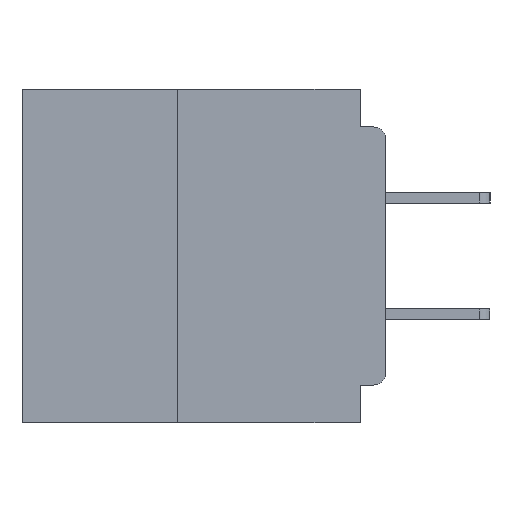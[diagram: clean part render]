
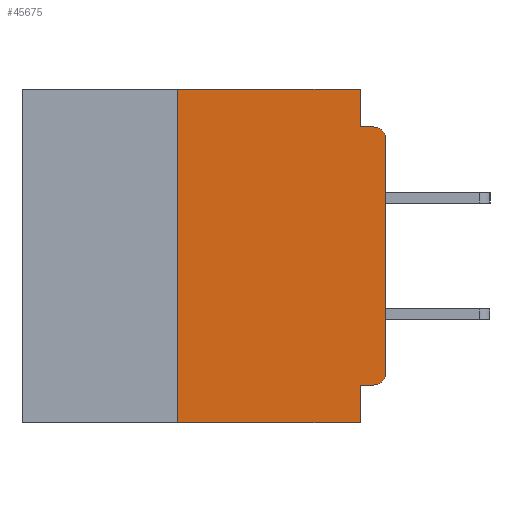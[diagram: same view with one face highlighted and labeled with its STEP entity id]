
A CAD part, left-side view. The second image highlights one B-rep face of the part: STEP entity #45675.
In plain terms, the highlighted planar face has unit normal (-1, 0, 0).
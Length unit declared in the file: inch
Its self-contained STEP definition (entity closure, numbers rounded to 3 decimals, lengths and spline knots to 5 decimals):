
#1313 = EDGE_CURVE ( 'NONE', #10483, #32483, #4898, .T. ) ;
#1629 = EDGE_CURVE ( 'NONE', #41125, #41036, #31239, .T. ) ;
#1631 = VERTEX_POINT ( 'NONE', #34603 ) ;
#1679 = ORIENTED_EDGE ( 'NONE', *, *, #33800, .F. ) ;
#1743 = CARTESIAN_POINT ( 'NONE',  ( 0., 0.031, 0. ) ) ;
#3261 = CARTESIAN_POINT ( 'NONE',  ( 0., 0.437, 0. ) ) ;
#3358 = ORIENTED_EDGE ( 'NONE', *, *, #36397, .F. ) ;
#4329 = CARTESIAN_POINT ( 'NONE',  ( 0., 0.437, 0. ) ) ;
#4350 = LINE ( 'NONE', #23653, #24455 ) ;
#4898 = LINE ( 'NONE', #48186, #14319 ) ;
#7079 = VECTOR ( 'NONE', #47031, 39.37008 ) ;
#7369 = LINE ( 'NONE', #23698, #26192 ) ;
#8332 = LINE ( 'NONE', #51061, #7079 ) ;
#8676 = CARTESIAN_POINT ( 'NONE',  ( 0., 0.015, -0.06 ) ) ;
#8730 = CARTESIAN_POINT ( 'NONE',  ( 0., 0.437, -0.4 ) ) ;
#10483 = VERTEX_POINT ( 'NONE', #18383 ) ;
#11990 = VECTOR ( 'NONE', #31342, 39.37008 ) ;
#12399 = PLANE ( 'NONE',  #33347 ) ;
#12697 = DIRECTION ( 'NONE',  ( 0., 0., -1. ) ) ;
#14319 = VECTOR ( 'NONE', #48076, 39.37008 ) ;
#14475 = CARTESIAN_POINT ( 'NONE',  ( 0., 0., 0. ) ) ;
#15382 = ORIENTED_EDGE ( 'NONE', *, *, #1629, .T. ) ;
#16089 = CARTESIAN_POINT ( 'NONE',  ( 0., 0.031, 0. ) ) ;
#16439 = DIRECTION ( 'NONE',  ( 0., 0., -1. ) ) ;
#16702 = CARTESIAN_POINT ( 'NONE',  ( 0., 0.031, -0.045 ) ) ;
#17888 = VECTOR ( 'NONE', #22523, 39.37008 ) ;
#18383 = CARTESIAN_POINT ( 'NONE',  ( 0., 0.25, -0.4 ) ) ;
#18413 = ORIENTED_EDGE ( 'NONE', *, *, #25655, .F. ) ;
#18552 = VERTEX_POINT ( 'NONE', #1743 ) ;
#19575 = CARTESIAN_POINT ( 'NONE',  ( 0., 0.25, 0. ) ) ;
#21410 = LINE ( 'NONE', #3261, #11990 ) ;
#21586 = ORIENTED_EDGE ( 'NONE', *, *, #1313, .F. ) ;
#22523 = DIRECTION ( 'NONE',  ( 0., 0., 1. ) ) ;
#23374 = VERTEX_POINT ( 'NONE', #36305 ) ;
#23653 = CARTESIAN_POINT ( 'NONE',  ( 0., 0.031, -0.4 ) ) ;
#23698 = CARTESIAN_POINT ( 'NONE',  ( 0., 0., -0.355 ) ) ;
#24372 = ORIENTED_EDGE ( 'NONE', *, *, #35073, .T. ) ;
#24425 = VECTOR ( 'NONE', #32782, 39.37008 ) ;
#24455 = VECTOR ( 'NONE', #27669, 39.37008 ) ;
#24699 = AXIS2_PLACEMENT_3D ( 'NONE', #33983, #33919, #33802 ) ;
#25389 = FACE_OUTER_BOUND ( 'NONE', #36045, .T. ) ;
#25655 = EDGE_CURVE ( 'NONE', #32483, #18552, #21410, .T. ) ;
#25910 = VECTOR ( 'NONE', #36122, 39.37008 ) ;
#26192 = VECTOR ( 'NONE', #47794, 39.37008 ) ;
#26659 = EDGE_CURVE ( 'NONE', #43019, #23374, #4350, .T. ) ;
#27158 = LINE ( 'NONE', #16089, #25910 ) ;
#27378 = AXIS2_PLACEMENT_3D ( 'NONE', #8676, #36779, #12697 ) ;
#27669 = DIRECTION ( 'NONE',  ( 0., 0., -1. ) ) ;
#27868 = CARTESIAN_POINT ( 'NONE',  ( 0., 0., -0.34 ) ) ;
#28113 = CARTESIAN_POINT ( 'NONE',  ( 0., 0., -0.06 ) ) ;
#30764 = ORIENTED_EDGE ( 'NONE', *, *, #49836, .T. ) ;
#31239 = CIRCLE ( 'NONE', #24699, 0.015 ) ;
#31342 = DIRECTION ( 'NONE',  ( 0., -1., 0. ) ) ;
#32483 = VERTEX_POINT ( 'NONE', #19575 ) ;
#32782 = DIRECTION ( 'NONE',  ( 0., -1., 0. ) ) ;
#33170 = CARTESIAN_POINT ( 'NONE',  ( 0., 0.031, -0.355 ) ) ;
#33347 = AXIS2_PLACEMENT_3D ( 'NONE', #4329, #40495, #16439 ) ;
#33800 = EDGE_CURVE ( 'NONE', #41125, #43019, #7369, .T. ) ;
#33802 = DIRECTION ( 'NONE',  ( 0., 0., -1. ) ) ;
#33849 = VERTEX_POINT ( 'NONE', #16702 ) ;
#33919 = DIRECTION ( 'NONE',  ( -1., 0., 0. ) ) ;
#33983 = CARTESIAN_POINT ( 'NONE',  ( 0., 0.015, -0.34 ) ) ;
#34603 = CARTESIAN_POINT ( 'NONE',  ( 0., 0.015, -0.045 ) ) ;
#35073 = EDGE_CURVE ( 'NONE', #41036, #51634, #39267, .T. ) ;
#36045 = EDGE_LOOP ( 'NONE', ( #24372, #30764, #3358, #39801, #18413, #21586, #37112, #46084, #1679, #15382 ) ) ;
#36122 = DIRECTION ( 'NONE',  ( 0., 0., -1. ) ) ;
#36305 = CARTESIAN_POINT ( 'NONE',  ( 0., 0.031, -0.4 ) ) ;
#36371 = LINE ( 'NONE', #8730, #24425 ) ;
#36397 = EDGE_CURVE ( 'NONE', #33849, #1631, #8332, .T. ) ;
#36779 = DIRECTION ( 'NONE',  ( -1., 0., 0. ) ) ;
#37112 = ORIENTED_EDGE ( 'NONE', *, *, #48547, .T. ) ;
#39267 = LINE ( 'NONE', #14475, #17888 ) ;
#39801 = ORIENTED_EDGE ( 'NONE', *, *, #45632, .F. ) ;
#40495 = DIRECTION ( 'NONE',  ( 1., 0., 0. ) ) ;
#41036 = VERTEX_POINT ( 'NONE', #27868 ) ;
#41125 = VERTEX_POINT ( 'NONE', #44402 ) ;
#43019 = VERTEX_POINT ( 'NONE', #33170 ) ;
#44402 = CARTESIAN_POINT ( 'NONE',  ( 0., 0.015, -0.355 ) ) ;
#45632 = EDGE_CURVE ( 'NONE', #18552, #33849, #27158, .T. ) ;
#45675 = ADVANCED_FACE ( 'NONE', ( #25389 ), #12399, .F. ) ;
#46084 = ORIENTED_EDGE ( 'NONE', *, *, #26659, .F. ) ;
#47031 = DIRECTION ( 'NONE',  ( 0., -1., 0. ) ) ;
#47794 = DIRECTION ( 'NONE',  ( 0., 1., 0. ) ) ;
#48076 = DIRECTION ( 'NONE',  ( 0., 0., 1. ) ) ;
#48186 = CARTESIAN_POINT ( 'NONE',  ( 0., 0.25, -0.4 ) ) ;
#48196 = CIRCLE ( 'NONE', #27378, 0.015 ) ;
#48547 = EDGE_CURVE ( 'NONE', #10483, #23374, #36371, .T. ) ;
#49836 = EDGE_CURVE ( 'NONE', #51634, #1631, #48196, .T. ) ;
#51061 = CARTESIAN_POINT ( 'NONE',  ( 0., 0., -0.045 ) ) ;
#51634 = VERTEX_POINT ( 'NONE', #28113 ) ;
